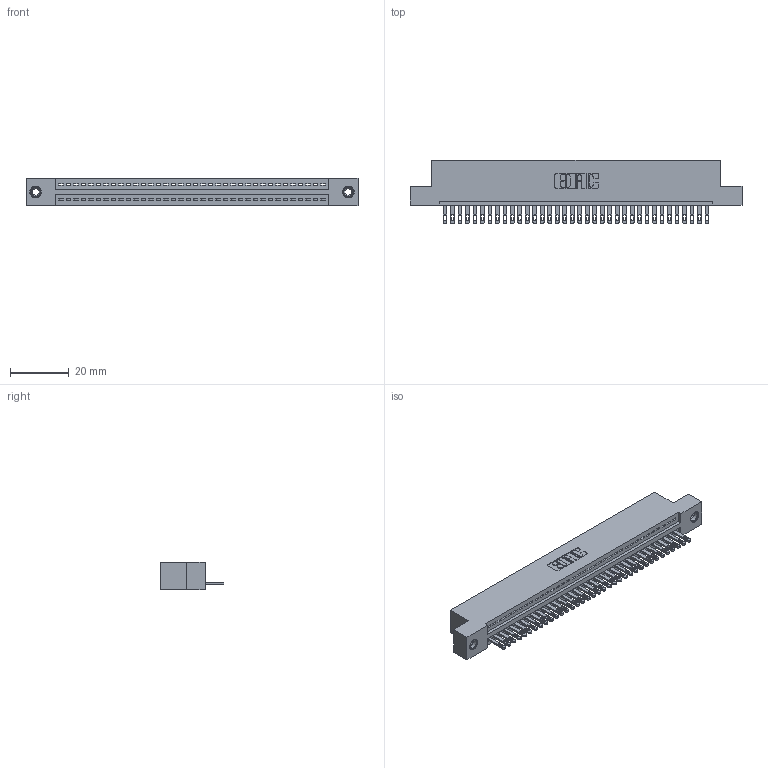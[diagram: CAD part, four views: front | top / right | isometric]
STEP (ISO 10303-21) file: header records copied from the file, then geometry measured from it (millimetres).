
FILE_DESCRIPTION (( 'STEP AP203' ), '1' );
FILE_NAME ('345-036-500-108.STEP', '2018-08-29T08:20:10', ( '' ), ( '' ), 'SwSTEP 2.0', 'SolidWorks 2016', '' );
FILE_SCHEMA (( 'CONFIG_CONTROL_DESIGN' ));
Length unit declared in the file: inch
Products named in the file (4): 345-292-001_345-293-100; 345-250-001_345-250-003-102; 345-036-500-108; 345 Part_Flush Mounting Lugs - 0.156 Dia-TI
Assembly tree (39 placements, depth 2):
  345-036-500-108
    345 Part_Flush Mounting Lugs - 0.156 Dia-TI
    345-292-001_345-293-100  x36
    345-250-001_345-250-003-102  x2
Bounding box: 112.65 x 21.51 x 9.4 mm (x, y, z)
Volume: 10666.1 mm3; surface area: 14192.8 mm2
Topology: 39 solids, 39 shells, 2130 faces, 6525 edges, 4342 vertices
Faces by surface type: plane 1336, cylinder 778, cone 12, torus 4
Entity records: 29018 total; most frequent: CARTESIAN_POINT 5007, ORIENTED_EDGE 4970, DIRECTION 4411, EDGE_CURVE 2485, VECTOR 2185, LINE 2185, VERTEX_POINT 1652, AXIS2_PLACEMENT_3D 1113
